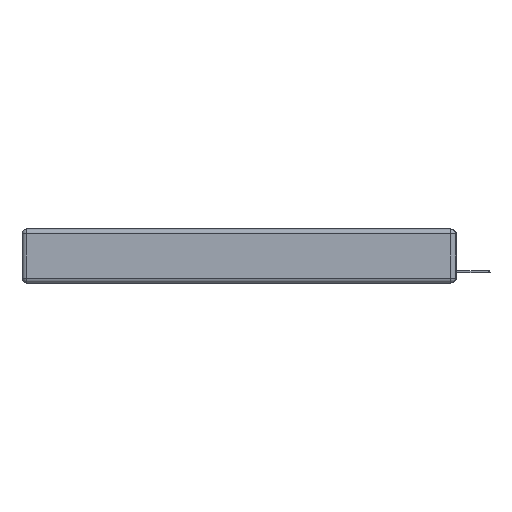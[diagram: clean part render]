
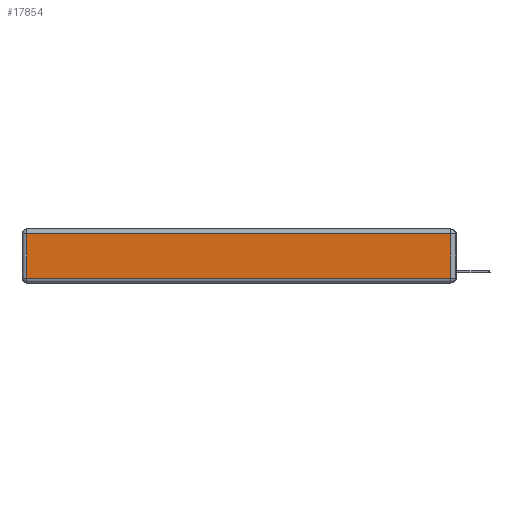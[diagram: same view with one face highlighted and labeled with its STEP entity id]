
A CAD part, left-side view. The second image highlights one B-rep face of the part: STEP entity #17854.
In plain terms, the highlighted planar face has unit normal (-1, 0, 0).
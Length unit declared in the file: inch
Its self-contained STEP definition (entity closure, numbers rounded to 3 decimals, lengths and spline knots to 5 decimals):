
#1305 = CARTESIAN_POINT ( 'NONE',  ( 0., 0.03, -0.313 ) ) ;
#1761 = VECTOR ( 'NONE', #20176, 39.37008 ) ;
#2507 = LINE ( 'NONE', #18895, #19451 ) ;
#3126 = DIRECTION ( 'NONE',  ( 0., 0., -1. ) ) ;
#3639 = PLANE ( 'NONE',  #13847 ) ;
#4240 = VERTEX_POINT ( 'NONE', #22914 ) ;
#5039 = EDGE_CURVE ( 'NONE', #24509, #4240, #16392, .T. ) ;
#5562 = DIRECTION ( 'NONE',  ( -1., 0., 0. ) ) ;
#6496 = FACE_OUTER_BOUND ( 'NONE', #11060, .T. ) ;
#7066 = VECTOR ( 'NONE', #23797, 39.37008 ) ;
#7176 = EDGE_CURVE ( 'NONE', #7738, #24509, #23371, .T. ) ;
#7423 = EDGE_CURVE ( 'NONE', #12094, #7738, #18097, .T. ) ;
#7626 = CARTESIAN_POINT ( 'NONE',  ( 0., 0., -0.343 ) ) ;
#7738 = VERTEX_POINT ( 'NONE', #1305 ) ;
#7812 = DIRECTION ( 'NONE',  ( 0., 1., 0. ) ) ;
#10543 = ORIENTED_EDGE ( 'NONE', *, *, #5039, .T. ) ;
#11060 = EDGE_LOOP ( 'NONE', ( #12424, #12957, #10543, #13386 ) ) ;
#11793 = CARTESIAN_POINT ( 'NONE',  ( 0., 0.03, -0.343 ) ) ;
#12094 = VERTEX_POINT ( 'NONE', #16444 ) ;
#12424 = ORIENTED_EDGE ( 'NONE', *, *, #7423, .T. ) ;
#12957 = ORIENTED_EDGE ( 'NONE', *, *, #7176, .T. ) ;
#13386 = ORIENTED_EDGE ( 'NONE', *, *, #22476, .T. ) ;
#13790 = CARTESIAN_POINT ( 'NONE',  ( 0., 0., -0.313 ) ) ;
#13847 = AXIS2_PLACEMENT_3D ( 'NONE', #7626, #5562, #23381 ) ;
#16392 = LINE ( 'NONE', #17265, #22871 ) ;
#16444 = CARTESIAN_POINT ( 'NONE',  ( 0., 2.72, -0.313 ) ) ;
#17265 = CARTESIAN_POINT ( 'NONE',  ( 0., 2.75, -0.03 ) ) ;
#17854 = ADVANCED_FACE ( 'NONE', ( #6496 ), #3639, .T. ) ;
#18097 = LINE ( 'NONE', #13790, #1761 ) ;
#18895 = CARTESIAN_POINT ( 'NONE',  ( 0., 2.72, -0.343 ) ) ;
#19451 = VECTOR ( 'NONE', #3126, 39.37008 ) ;
#20176 = DIRECTION ( 'NONE',  ( 0., -1., 0. ) ) ;
#20712 = CARTESIAN_POINT ( 'NONE',  ( 0., 0.03, -0.03 ) ) ;
#22476 = EDGE_CURVE ( 'NONE', #4240, #12094, #2507, .T. ) ;
#22871 = VECTOR ( 'NONE', #7812, 39.37008 ) ;
#22914 = CARTESIAN_POINT ( 'NONE',  ( 0., 2.72, -0.03 ) ) ;
#23371 = LINE ( 'NONE', #11793, #7066 ) ;
#23381 = DIRECTION ( 'NONE',  ( 0., 0., 1. ) ) ;
#23797 = DIRECTION ( 'NONE',  ( 0., 0., 1. ) ) ;
#24509 = VERTEX_POINT ( 'NONE', #20712 ) ;
